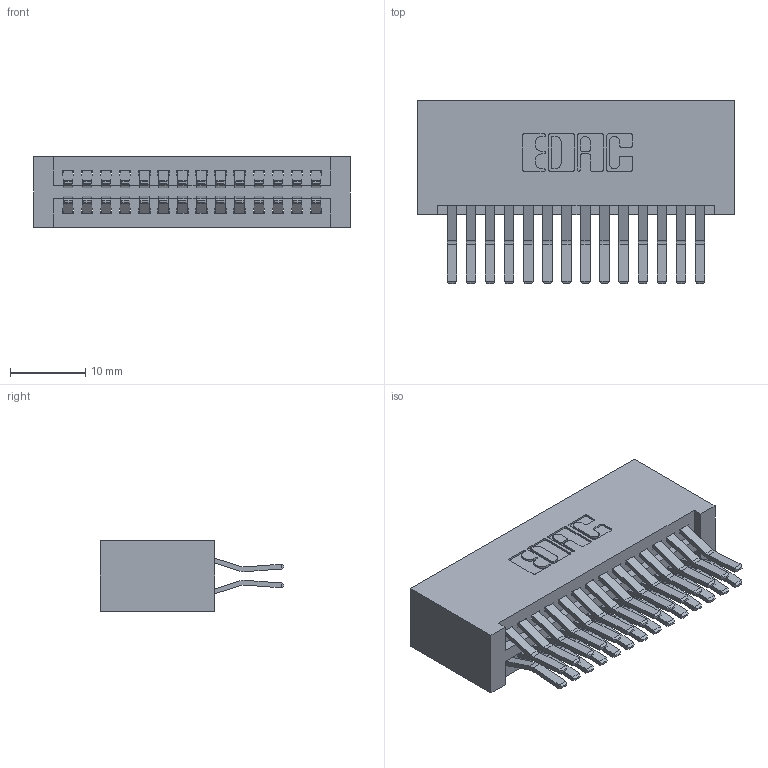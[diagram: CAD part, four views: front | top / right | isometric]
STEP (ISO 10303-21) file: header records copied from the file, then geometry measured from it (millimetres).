
FILE_DESCRIPTION (( 'STEP AP203' ), '1' );
FILE_NAME ('395-028-560-201.STEP', '2019-10-16T20:34:47', ( '' ), ( '' ), 'SwSTEP 2.0', 'SolidWorks 2016', '' );
FILE_SCHEMA (( 'CONFIG_CONTROL_DESIGN' ));
Length unit declared in the file: inch
Products named in the file (3): 345 Part_No Mounting Lugs; 345-292-001_560 Tail; 395-028-560-201
Assembly tree (29 placements, depth 2):
  395-028-560-201
    345 Part_No Mounting Lugs
    345-292-001_560 Tail  x28
Bounding box: 42.16 x 24.45 x 9.4 mm (x, y, z)
Volume: 4635.4 mm3; surface area: 7084.9 mm2
Topology: 29 solids, 29 shells, 1574 faces, 4657 edges, 3066 vertices
Faces by surface type: plane 1000, cylinder 574
Entity records: 14565 total; most frequent: CARTESIAN_POINT 2468, ORIENTED_EDGE 2402, DIRECTION 2209, EDGE_CURVE 1201, LINE 1017, VECTOR 1017, VERTEX_POINT 798, AXIS2_PLACEMENT_3D 596
